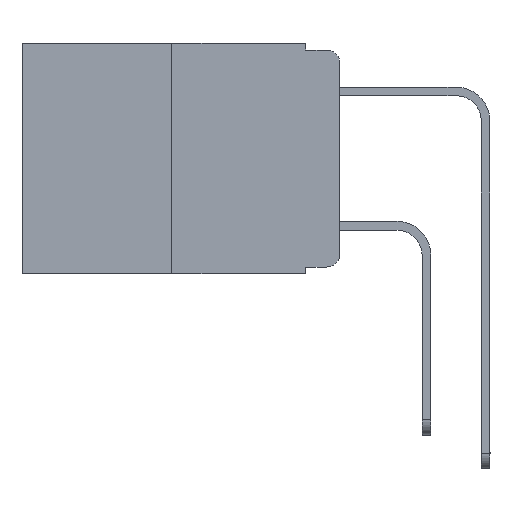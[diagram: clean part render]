
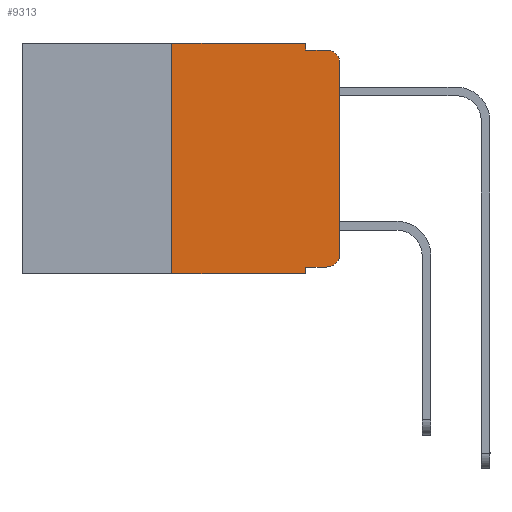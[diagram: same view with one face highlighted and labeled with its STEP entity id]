
A CAD part, left-side view. The second image highlights one B-rep face of the part: STEP entity #9313.
In plain terms, the highlighted planar face has unit normal (-1, 0, 0).
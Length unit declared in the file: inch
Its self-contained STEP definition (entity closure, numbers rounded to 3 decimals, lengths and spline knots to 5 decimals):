
#23 = VERTEX_POINT ( 'NONE', #8308 ) ;
#104 = DIRECTION ( 'NONE',  ( 0., -1., 0. ) ) ;
#318 = DIRECTION ( 'NONE',  ( 0., 0., -1. ) ) ;
#367 = ORIENTED_EDGE ( 'NONE', *, *, #2862, .F. ) ;
#521 = FACE_OUTER_BOUND ( 'NONE', #11358, .T. ) ;
#744 = EDGE_CURVE ( 'NONE', #8506, #989, #6144, .T. ) ;
#894 = VERTEX_POINT ( 'NONE', #7333 ) ;
#989 = VERTEX_POINT ( 'NONE', #8945 ) ;
#1674 = DIRECTION ( 'NONE',  ( -1., 0., 0. ) ) ;
#1791 = ORIENTED_EDGE ( 'NONE', *, *, #5670, .T. ) ;
#1870 = ORIENTED_EDGE ( 'NONE', *, *, #744, .F. ) ;
#1968 = CIRCLE ( 'NONE', #3307, 0.02 ) ;
#2172 = LINE ( 'NONE', #6464, #8770 ) ;
#2175 = LINE ( 'NONE', #6531, #13293 ) ;
#2241 = AXIS2_PLACEMENT_3D ( 'NONE', #7092, #7023, #11401 ) ;
#2352 = VECTOR ( 'NONE', #318, 39.37008 ) ;
#2702 = ORIENTED_EDGE ( 'NONE', *, *, #8625, .T. ) ;
#2862 = EDGE_CURVE ( 'NONE', #13420, #894, #7462, .T. ) ;
#2898 = VECTOR ( 'NONE', #10733, 39.37008 ) ;
#3307 = AXIS2_PLACEMENT_3D ( 'NONE', #13343, #8880, #7825 ) ;
#3723 = VECTOR ( 'NONE', #6689, 39.37008 ) ;
#3727 = CARTESIAN_POINT ( 'NONE',  ( 0., 0.473, -0.343 ) ) ;
#3815 = EDGE_CURVE ( 'NONE', #13420, #8826, #5776, .T. ) ;
#3853 = VERTEX_POINT ( 'NONE', #13403 ) ;
#4174 = CARTESIAN_POINT ( 'NONE',  ( 0., 0.25, 0. ) ) ;
#4380 = VERTEX_POINT ( 'NONE', #8228 ) ;
#4454 = CARTESIAN_POINT ( 'NONE',  ( 0., 0.02, -0.333 ) ) ;
#4734 = ORIENTED_EDGE ( 'NONE', *, *, #9986, .T. ) ;
#4781 = LINE ( 'NONE', #3727, #5652 ) ;
#5020 = ORIENTED_EDGE ( 'NONE', *, *, #3815, .T. ) ;
#5230 = CARTESIAN_POINT ( 'NONE',  ( 0., 0., 0. ) ) ;
#5527 = VERTEX_POINT ( 'NONE', #4174 ) ;
#5652 = VECTOR ( 'NONE', #6055, 39.37008 ) ;
#5670 = EDGE_CURVE ( 'NONE', #23, #989, #1968, .T. ) ;
#5681 = VERTEX_POINT ( 'NONE', #6833 ) ;
#5776 = LINE ( 'NONE', #5844, #3723 ) ;
#5844 = CARTESIAN_POINT ( 'NONE',  ( 0., 0.051, -0.333 ) ) ;
#5963 = DIRECTION ( 'NONE',  ( 0., 0., -1. ) ) ;
#6036 = CARTESIAN_POINT ( 'NONE',  ( 0., 0.02, -0.313 ) ) ;
#6055 = DIRECTION ( 'NONE',  ( 0., -1., 0. ) ) ;
#6144 = LINE ( 'NONE', #9241, #13421 ) ;
#6306 = AXIS2_PLACEMENT_3D ( 'NONE', #6036, #1674, #5963 ) ;
#6464 = CARTESIAN_POINT ( 'NONE',  ( 0., 0.473, 0. ) ) ;
#6531 = CARTESIAN_POINT ( 'NONE',  ( 0., 0.051, 0. ) ) ;
#6689 = DIRECTION ( 'NONE',  ( 0., -1., 0. ) ) ;
#6833 = CARTESIAN_POINT ( 'NONE',  ( 0., 0.25, -0.343 ) ) ;
#7023 = DIRECTION ( 'NONE',  ( 1., 0., 0. ) ) ;
#7092 = CARTESIAN_POINT ( 'NONE',  ( 0., 0.473, 0. ) ) ;
#7333 = CARTESIAN_POINT ( 'NONE',  ( 0., 0.051, -0.343 ) ) ;
#7462 = LINE ( 'NONE', #8650, #2352 ) ;
#7825 = DIRECTION ( 'NONE',  ( 0., 0., -1. ) ) ;
#8023 = CARTESIAN_POINT ( 'NONE',  ( 0., 0.25, 0. ) ) ;
#8173 = LINE ( 'NONE', #8023, #8993 ) ;
#8228 = CARTESIAN_POINT ( 'NONE',  ( 0., 0.051, 0. ) ) ;
#8308 = CARTESIAN_POINT ( 'NONE',  ( 0., 0., -0.03 ) ) ;
#8506 = VERTEX_POINT ( 'NONE', #13963 ) ;
#8625 = EDGE_CURVE ( 'NONE', #3853, #23, #9389, .T. ) ;
#8650 = CARTESIAN_POINT ( 'NONE',  ( 0., 0.051, 0. ) ) ;
#8770 = VECTOR ( 'NONE', #104, 39.37008 ) ;
#8826 = VERTEX_POINT ( 'NONE', #4454 ) ;
#8831 = ORIENTED_EDGE ( 'NONE', *, *, #11261, .F. ) ;
#8880 = DIRECTION ( 'NONE',  ( -1., 0., 0. ) ) ;
#8945 = CARTESIAN_POINT ( 'NONE',  ( 0., 0.02, -0.01 ) ) ;
#8993 = VECTOR ( 'NONE', #12531, 39.37008 ) ;
#9241 = CARTESIAN_POINT ( 'NONE',  ( 0., 0.051, -0.01 ) ) ;
#9313 = ADVANCED_FACE ( 'NONE', ( #521 ), #12454, .F. ) ;
#9315 = ORIENTED_EDGE ( 'NONE', *, *, #11638, .F. ) ;
#9378 = DIRECTION ( 'NONE',  ( 0., -1., 0. ) ) ;
#9389 = LINE ( 'NONE', #5230, #2898 ) ;
#9670 = EDGE_CURVE ( 'NONE', #5527, #4380, #2172, .T. ) ;
#9986 = EDGE_CURVE ( 'NONE', #8826, #3853, #11485, .T. ) ;
#10733 = DIRECTION ( 'NONE',  ( 0., 0., 1. ) ) ;
#10823 = CARTESIAN_POINT ( 'NONE',  ( 0., 0.051, -0.333 ) ) ;
#11261 = EDGE_CURVE ( 'NONE', #5681, #5527, #8173, .T. ) ;
#11358 = EDGE_LOOP ( 'NONE', ( #2702, #1791, #1870, #9315, #13203, #8831, #13486, #367, #5020, #4734 ) ) ;
#11401 = DIRECTION ( 'NONE',  ( 0., 0., -1. ) ) ;
#11485 = CIRCLE ( 'NONE', #6306, 0.02 ) ;
#11638 = EDGE_CURVE ( 'NONE', #4380, #8506, #2175, .T. ) ;
#12454 = PLANE ( 'NONE',  #2241 ) ;
#12531 = DIRECTION ( 'NONE',  ( 0., 0., 1. ) ) ;
#12653 = EDGE_CURVE ( 'NONE', #5681, #894, #4781, .T. ) ;
#13203 = ORIENTED_EDGE ( 'NONE', *, *, #9670, .F. ) ;
#13293 = VECTOR ( 'NONE', #13583, 39.37008 ) ;
#13343 = CARTESIAN_POINT ( 'NONE',  ( 0., 0.02, -0.03 ) ) ;
#13403 = CARTESIAN_POINT ( 'NONE',  ( 0., 0., -0.313 ) ) ;
#13420 = VERTEX_POINT ( 'NONE', #10823 ) ;
#13421 = VECTOR ( 'NONE', #9378, 39.37008 ) ;
#13486 = ORIENTED_EDGE ( 'NONE', *, *, #12653, .T. ) ;
#13583 = DIRECTION ( 'NONE',  ( 0., 0., -1. ) ) ;
#13963 = CARTESIAN_POINT ( 'NONE',  ( 0., 0.051, -0.01 ) ) ;
